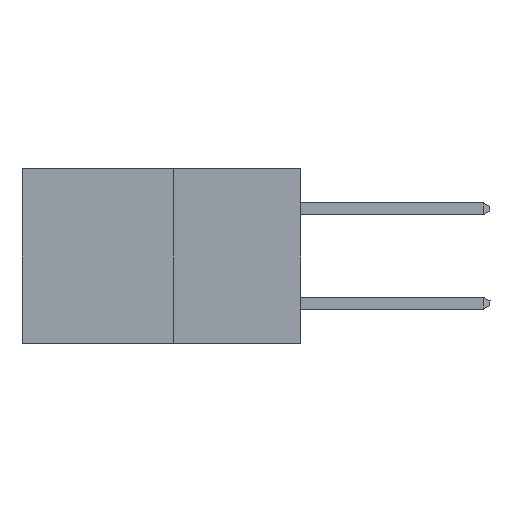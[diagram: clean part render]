
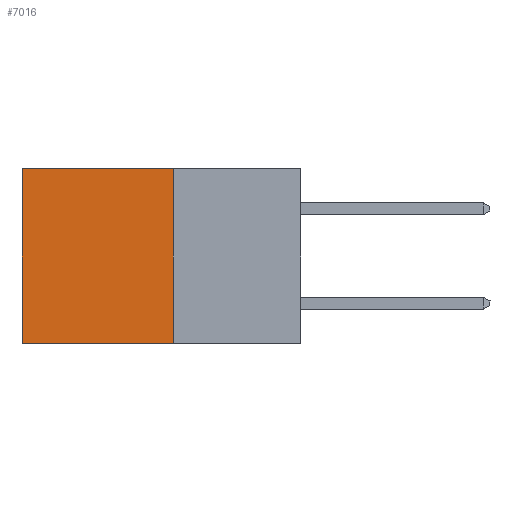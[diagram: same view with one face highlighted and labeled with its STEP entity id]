
A CAD part, left-side view. The second image highlights one B-rep face of the part: STEP entity #7016.
In plain terms, the highlighted planar face has unit normal (-1, 0, 0).
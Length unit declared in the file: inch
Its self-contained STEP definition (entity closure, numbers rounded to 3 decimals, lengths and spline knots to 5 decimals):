
#595 = DIRECTION ( 'NONE',  ( 0., 0., -1. ) ) ;
#624 = DIRECTION ( 'NONE',  ( 1., 0., 0. ) ) ;
#670 = CARTESIAN_POINT ( 'NONE',  ( 0.277, 0.27, -0.37 ) ) ;
#774 = PLANE ( 'NONE',  #1892 ) ;
#1892 = AXIS2_PLACEMENT_3D ( 'NONE', #670, #624, #595 ) ;
#4098 = LINE ( 'NONE', #11128, #20144 ) ;
#4273 = EDGE_CURVE ( 'NONE', #6587, #4528, #4098, .T. ) ;
#4418 = CARTESIAN_POINT ( 'NONE',  ( 0.277, 0.27, -0.37 ) ) ;
#4528 = VERTEX_POINT ( 'NONE', #5297 ) ;
#4936 = EDGE_CURVE ( 'NONE', #17077, #4528, #16542, .T. ) ;
#5142 = ORIENTED_EDGE ( 'NONE', *, *, #4273, .F. ) ;
#5297 = CARTESIAN_POINT ( 'NONE',  ( 0.277, 0.59, -0.37 ) ) ;
#5383 = CARTESIAN_POINT ( 'NONE',  ( 0.277, 0.27, -0.37 ) ) ;
#5925 = CARTESIAN_POINT ( 'NONE',  ( 0.277, 0.59, 0. ) ) ;
#6587 = VERTEX_POINT ( 'NONE', #4418 ) ;
#6855 = VECTOR ( 'NONE', #10412, 39.37008 ) ;
#7016 = ADVANCED_FACE ( 'NONE', ( #16280 ), #774, .F. ) ;
#7490 = VECTOR ( 'NONE', #19104, 39.37008 ) ;
#8243 = EDGE_LOOP ( 'NONE', ( #20412, #5142, #16416, #10775 ) ) ;
#8614 = CARTESIAN_POINT ( 'NONE',  ( 0.277, 0.27, 0. ) ) ;
#8883 = CARTESIAN_POINT ( 'NONE',  ( 0.277, 0.27, 0. ) ) ;
#10412 = DIRECTION ( 'NONE',  ( 0., 0., -1. ) ) ;
#10557 = DIRECTION ( 'NONE',  ( 0., 1., 0. ) ) ;
#10682 = LINE ( 'NONE', #8883, #18559 ) ;
#10775 = ORIENTED_EDGE ( 'NONE', *, *, #11215, .T. ) ;
#11128 = CARTESIAN_POINT ( 'NONE',  ( 0.277, 0.27, -0.37 ) ) ;
#11215 = EDGE_CURVE ( 'NONE', #17214, #17077, #10682, .T. ) ;
#11262 = LINE ( 'NONE', #5383, #6855 ) ;
#11403 = DIRECTION ( 'NONE',  ( 0., 1., 0. ) ) ;
#16280 = FACE_OUTER_BOUND ( 'NONE', #8243, .T. ) ;
#16416 = ORIENTED_EDGE ( 'NONE', *, *, #17747, .F. ) ;
#16542 = LINE ( 'NONE', #19086, #7490 ) ;
#17077 = VERTEX_POINT ( 'NONE', #5925 ) ;
#17214 = VERTEX_POINT ( 'NONE', #8614 ) ;
#17747 = EDGE_CURVE ( 'NONE', #17214, #6587, #11262, .T. ) ;
#18559 = VECTOR ( 'NONE', #10557, 39.37008 ) ;
#19086 = CARTESIAN_POINT ( 'NONE',  ( 0.277, 0.59, -0.37 ) ) ;
#19104 = DIRECTION ( 'NONE',  ( 0., 0., -1. ) ) ;
#20144 = VECTOR ( 'NONE', #11403, 39.37008 ) ;
#20412 = ORIENTED_EDGE ( 'NONE', *, *, #4936, .T. ) ;
